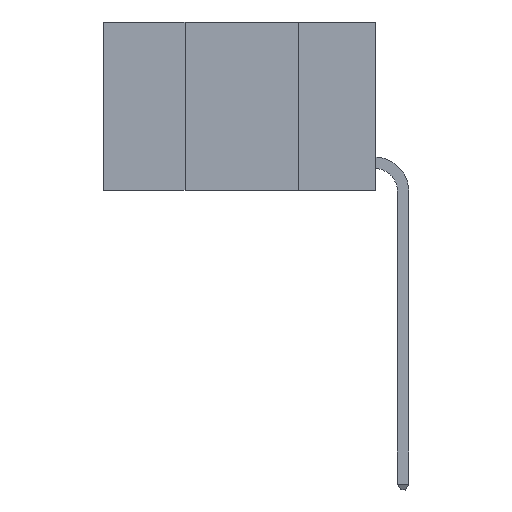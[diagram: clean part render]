
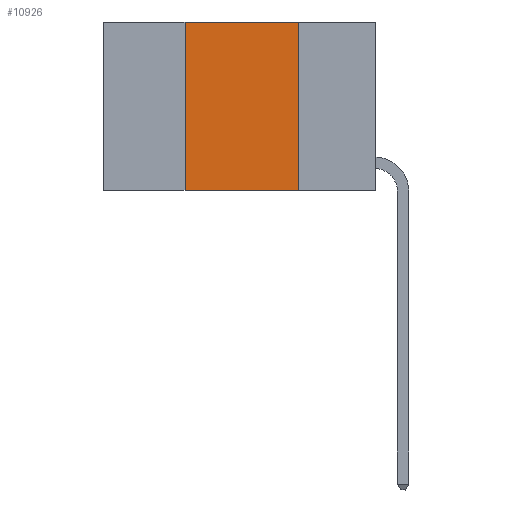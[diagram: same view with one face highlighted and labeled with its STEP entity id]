
A CAD part, left-side view. The second image highlights one B-rep face of the part: STEP entity #10926.
In plain terms, the highlighted planar face has unit normal (-1, 0, 0).
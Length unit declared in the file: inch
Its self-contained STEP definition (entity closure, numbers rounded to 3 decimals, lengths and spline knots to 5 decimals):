
#123 = DIRECTION ( 'NONE',  ( 0., 0., 1. ) ) ;
#1234 = PLANE ( 'NONE',  #5790 ) ;
#1237 = CARTESIAN_POINT ( 'NONE',  ( 0., 0.42, 0. ) ) ;
#1344 = CARTESIAN_POINT ( 'NONE',  ( 0., 0.6, 0. ) ) ;
#1838 = VERTEX_POINT ( 'NONE', #11896 ) ;
#2238 = EDGE_CURVE ( 'NONE', #1838, #7178, #8663, .T. ) ;
#2302 = VECTOR ( 'NONE', #123, 39.37008 ) ;
#2405 = DIRECTION ( 'NONE',  ( 1., 0., 0. ) ) ;
#2884 = VECTOR ( 'NONE', #6310, 39.37008 ) ;
#2912 = EDGE_LOOP ( 'NONE', ( #5525, #5836, #7474, #8056 ) ) ;
#4108 = CARTESIAN_POINT ( 'NONE',  ( 0., 0.17, -0.37 ) ) ;
#4358 = VERTEX_POINT ( 'NONE', #10128 ) ;
#5062 = EDGE_CURVE ( 'NONE', #1838, #12148, #5736, .T. ) ;
#5311 = CARTESIAN_POINT ( 'NONE',  ( 0., 0.6, -0.37 ) ) ;
#5525 = ORIENTED_EDGE ( 'NONE', *, *, #5745, .F. ) ;
#5736 = LINE ( 'NONE', #12813, #2302 ) ;
#5745 = EDGE_CURVE ( 'NONE', #4358, #7178, #11591, .T. ) ;
#5790 = AXIS2_PLACEMENT_3D ( 'NONE', #7542, #2405, #9589 ) ;
#5836 = ORIENTED_EDGE ( 'NONE', *, *, #5915, .F. ) ;
#5915 = EDGE_CURVE ( 'NONE', #12148, #4358, #12083, .T. ) ;
#6310 = DIRECTION ( 'NONE',  ( 0., -1., 0. ) ) ;
#6967 = VECTOR ( 'NONE', #9682, 39.37008 ) ;
#7178 = VERTEX_POINT ( 'NONE', #4108 ) ;
#7419 = DIRECTION ( 'NONE',  ( 0., 0., -1. ) ) ;
#7474 = ORIENTED_EDGE ( 'NONE', *, *, #5062, .F. ) ;
#7542 = CARTESIAN_POINT ( 'NONE',  ( 0., 0.6, 0. ) ) ;
#8056 = ORIENTED_EDGE ( 'NONE', *, *, #2238, .T. ) ;
#8663 = LINE ( 'NONE', #5311, #2884 ) ;
#9589 = DIRECTION ( 'NONE',  ( 0., 0., -1. ) ) ;
#9682 = DIRECTION ( 'NONE',  ( 0., -1., 0. ) ) ;
#10128 = CARTESIAN_POINT ( 'NONE',  ( 0., 0.17, 0. ) ) ;
#10926 = ADVANCED_FACE ( 'NONE', ( #13222 ), #1234, .F. ) ;
#11591 = LINE ( 'NONE', #12525, #11928 ) ;
#11896 = CARTESIAN_POINT ( 'NONE',  ( 0., 0.42, -0.37 ) ) ;
#11928 = VECTOR ( 'NONE', #7419, 39.37008 ) ;
#12083 = LINE ( 'NONE', #1344, #6967 ) ;
#12148 = VERTEX_POINT ( 'NONE', #1237 ) ;
#12525 = CARTESIAN_POINT ( 'NONE',  ( 0., 0.17, 0. ) ) ;
#12813 = CARTESIAN_POINT ( 'NONE',  ( 0., 0.42, 0. ) ) ;
#13222 = FACE_OUTER_BOUND ( 'NONE', #2912, .T. ) ;
